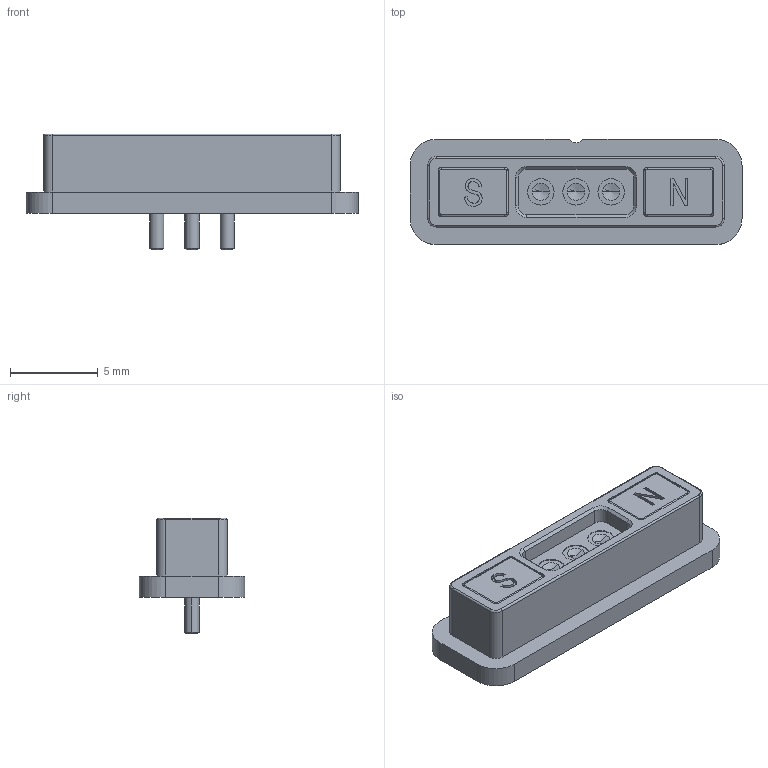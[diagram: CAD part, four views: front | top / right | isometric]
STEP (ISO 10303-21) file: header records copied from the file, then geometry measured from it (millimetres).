
FILE_DESCRIPTION (( 'STEP AP203' ), '1' );
FILE_NAME ('686-F0321250110.STEP', '2023-02-14T10:37:23', ( 'Magnum' ), ( '' ), 'SwSTEP 2.0', 'SolidWorks 2020', '' );
FILE_SCHEMA (( 'CONFIG_CONTROL_DESIGN' ));
Length unit declared in the file: millimetre
Products named in the file (1): 686-F0321250110
Bounding box: 18.9 x 6 x 6.6 mm (x, y, z)
Volume: 313 mm3; surface area: 539.9 mm2
Topology: 4 solids, 6 shells, 206 faces, 486 edges, 302 vertices
Faces by surface type: plane 82, cylinder 69, bspline 30, cone 21, torus 4
Entity records: 6836 total; most frequent: CARTESIAN_POINT 2059, DIRECTION 987, ORIENTED_EDGE 960, EDGE_CURVE 480, AXIS2_PLACEMENT_3D 358, VERTEX_POINT 302, LINE 271, VECTOR 271
